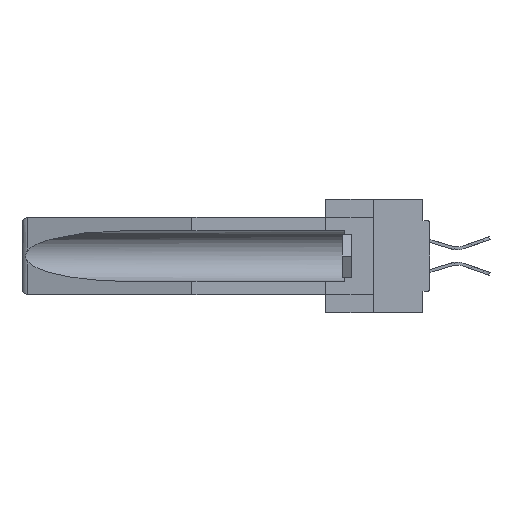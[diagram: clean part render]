
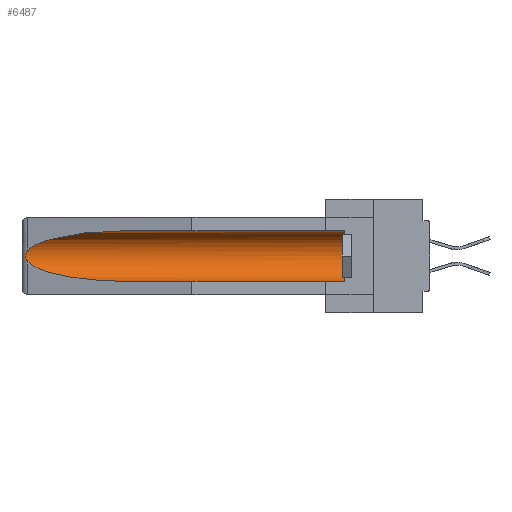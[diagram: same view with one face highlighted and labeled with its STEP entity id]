
A CAD part, left-side view. The second image highlights one B-rep face of the part: STEP entity #6487.
In plain terms, the highlighted cylindrical face has radius 2.857 mm (diameter 5.715 mm), a partial arc.
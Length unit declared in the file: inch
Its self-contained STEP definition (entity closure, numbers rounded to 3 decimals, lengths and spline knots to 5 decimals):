
#233 = DIRECTION ( 'NONE',  ( 0., 0., 1. ) ) ;
#448 = EDGE_CURVE ( 'NONE', #21810, #25098, #33990, .T. ) ;
#643 = AXIS2_PLACEMENT_3D ( 'NONE', #24292, #20641, #27301 ) ;
#2471 = EDGE_CURVE ( 'NONE', #10888, #29051, #32456, .T. ) ;
#2643 = CARTESIAN_POINT ( 'NONE',  ( 0.26597, 1.5296, -0.19026 ) ) ;
#3024 = FACE_OUTER_BOUND ( 'NONE', #21239, .T. ) ;
#4741 = ORIENTED_EDGE ( 'NONE', *, *, #6218, .T. ) ;
#5064 = CYLINDRICAL_SURFACE ( 'NONE', #643, 0.1125 ) ;
#5799 = ORIENTED_EDGE ( 'NONE', *, *, #23522, .T. ) ;
#6218 = EDGE_CURVE ( 'NONE', #25098, #35279, #26498, .T. ) ;
#6487 = ADVANCED_FACE ( 'NONE', ( #3024 ), #5064, .F. ) ;
#6595 = CARTESIAN_POINT ( 'NONE',  ( 0.155, 0.126, -0.1715 ) ) ;
#7663 = DIRECTION ( 'NONE',  ( 0., 1., 0. ) ) ;
#8105 =( BOUNDED_CURVE ( )  B_SPLINE_CURVE ( 3, ( #11566, #18052, #21028, #24553 ),
 .UNSPECIFIED., .F., .F. ) 
 B_SPLINE_CURVE_WITH_KNOTS ( ( 4, 4 ),
 ( 0.1948, 1.5708 ),
 .UNSPECIFIED. ) 
 CURVE ( )  GEOMETRIC_REPRESENTATION_ITEM ( )  RATIONAL_B_SPLINE_CURVE ( ( 1., 0.848, 0.848, 1. ) ) 
 REPRESENTATION_ITEM ( '' )  );
#8803 = VECTOR ( 'NONE', #15703, 39.37008 ) ;
#9533 = CARTESIAN_POINT ( 'NONE',  ( 0.21114, 1.30732, -0.059 ) ) ;
#9748 = CARTESIAN_POINT ( 'NONE',  ( 0.2673, 1.5327, -0.16383 ) ) ;
#10433 = CARTESIAN_POINT ( 'NONE',  ( 0.155, 1.07973, -0.284 ) ) ;
#10888 = VERTEX_POINT ( 'NONE', #34965 ) ;
#11566 = CARTESIAN_POINT ( 'NONE',  ( 0.26537, 1.52718, -0.19328 ) ) ;
#12365 = ORIENTED_EDGE ( 'NONE', *, *, #40446, .F. ) ;
#12978 = CARTESIAN_POINT ( 'NONE',  ( 0.26654, 1.53092, -0.15636 ) ) ;
#13144 = ORIENTED_EDGE ( 'NONE', *, *, #2471, .T. ) ;
#15538 = CARTESIAN_POINT ( 'NONE',  ( 0.2673, 1.53269, -0.17917 ) ) ;
#15703 = DIRECTION ( 'NONE',  ( 0., 1., 0. ) ) ;
#15817 = CARTESIAN_POINT ( 'NONE',  ( 0.26597, 1.52961, -0.15275 ) ) ;
#15879 = LINE ( 'NONE', #18674, #8803 ) ;
#18052 = CARTESIAN_POINT ( 'NONE',  ( 0.25451, 1.48313, -0.24835 ) ) ;
#18399 = VECTOR ( 'NONE', #7663, 39.37008 ) ;
#18674 = CARTESIAN_POINT ( 'NONE',  ( 0.155, -0.30754, -0.059 ) ) ;
#19268 = CARTESIAN_POINT ( 'NONE',  ( 0.25451, 1.48313, -0.09465 ) ) ;
#20641 = DIRECTION ( 'NONE',  ( 0., 1., 0. ) ) ;
#21028 = CARTESIAN_POINT ( 'NONE',  ( 0.21114, 1.30732, -0.284 ) ) ;
#21239 = EDGE_LOOP ( 'NONE', ( #22610, #4741, #38864, #12365, #13144, #5799 ) ) ;
#21810 = VERTEX_POINT ( 'NONE', #22755 ) ;
#22126 = EDGE_CURVE ( 'NONE', #35279, #29393, #8105, .T. ) ;
#22606 = CARTESIAN_POINT ( 'NONE',  ( 0.26537, 1.52718, -0.14972 ) ) ;
#22610 = ORIENTED_EDGE ( 'NONE', *, *, #448, .T. ) ;
#22755 = CARTESIAN_POINT ( 'NONE',  ( 0.155, 1.07973, -0.059 ) ) ;
#22756 = AXIS2_PLACEMENT_3D ( 'NONE', #6595, #38892, #233 ) ;
#23522 = EDGE_CURVE ( 'NONE', #29051, #21810, #15879, .T. ) ;
#24292 = CARTESIAN_POINT ( 'NONE',  ( 0.155, -0.30754, -0.1715 ) ) ;
#24553 = CARTESIAN_POINT ( 'NONE',  ( 0.155, 1.07973, -0.284 ) ) ;
#24734 = CARTESIAN_POINT ( 'NONE',  ( 0.155, 0.126, -0.059 ) ) ;
#25098 = VERTEX_POINT ( 'NONE', #36075 ) ;
#25306 = CARTESIAN_POINT ( 'NONE',  ( 0.26537, 1.52718, -0.19328 ) ) ;
#26498 = B_SPLINE_CURVE_WITH_KNOTS ( 'NONE', 3,
 ( #22606, #15817, #12978, #9748, #32366, #41751, #15538, #38078, #2643, #25306 ),
 .UNSPECIFIED., .F., .F.,
 ( 4, 2, 2, 2, 4 ),
 ( 0., 0.00029, 0.00058, 0.00087, 0.00117 ),
 .UNSPECIFIED. ) ;
#27032 = CARTESIAN_POINT ( 'NONE',  ( 0.155, -0.30754, -0.284 ) ) ;
#27301 = DIRECTION ( 'NONE',  ( 0., 0., 1. ) ) ;
#29051 = VERTEX_POINT ( 'NONE', #24734 ) ;
#29393 = VERTEX_POINT ( 'NONE', #10433 ) ;
#32366 = CARTESIAN_POINT ( 'NONE',  ( 0.2675, 1.53308, -0.16763 ) ) ;
#32456 = CIRCLE ( 'NONE', #22756, 0.1125 ) ;
#33990 =( BOUNDED_CURVE ( )  B_SPLINE_CURVE ( 3, ( #38136, #9533, #19268, #38000 ),
 .UNSPECIFIED., .F., .F. ) 
 B_SPLINE_CURVE_WITH_KNOTS ( ( 4, 4 ),
 ( 4.71239, 6.08839 ),
 .UNSPECIFIED. ) 
 CURVE ( )  GEOMETRIC_REPRESENTATION_ITEM ( )  RATIONAL_B_SPLINE_CURVE ( ( 1., 0.848, 0.848, 1. ) ) 
 REPRESENTATION_ITEM ( '' )  );
#34965 = CARTESIAN_POINT ( 'NONE',  ( 0.155, 0.126, -0.284 ) ) ;
#35279 = VERTEX_POINT ( 'NONE', #40861 ) ;
#36075 = CARTESIAN_POINT ( 'NONE',  ( 0.26537, 1.52718, -0.14972 ) ) ;
#38000 = CARTESIAN_POINT ( 'NONE',  ( 0.26537, 1.52718, -0.14972 ) ) ;
#38078 = CARTESIAN_POINT ( 'NONE',  ( 0.26655, 1.53094, -0.18657 ) ) ;
#38136 = CARTESIAN_POINT ( 'NONE',  ( 0.155, 1.07973, -0.059 ) ) ;
#38864 = ORIENTED_EDGE ( 'NONE', *, *, #22126, .T. ) ;
#38892 = DIRECTION ( 'NONE',  ( 0., -1., 0. ) ) ;
#39603 = LINE ( 'NONE', #27032, #18399 ) ;
#40446 = EDGE_CURVE ( 'NONE', #10888, #29393, #39603, .T. ) ;
#40861 = CARTESIAN_POINT ( 'NONE',  ( 0.26537, 1.52718, -0.19328 ) ) ;
#41751 = CARTESIAN_POINT ( 'NONE',  ( 0.2675, 1.53308, -0.17534 ) ) ;
